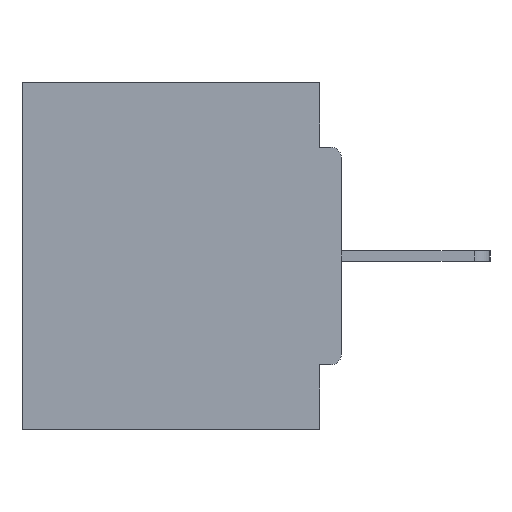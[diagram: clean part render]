
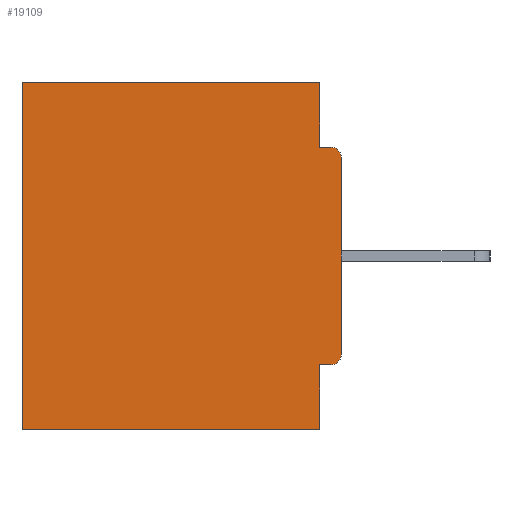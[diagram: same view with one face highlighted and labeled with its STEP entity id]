
A CAD part, left-side view. The second image highlights one B-rep face of the part: STEP entity #19109.
In plain terms, the highlighted planar face has unit normal (-1, 0, 0).
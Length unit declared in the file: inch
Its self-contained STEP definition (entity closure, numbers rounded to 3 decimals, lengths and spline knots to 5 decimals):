
#626 = LINE ( 'NONE', #946, #13052 ) ;
#946 = CARTESIAN_POINT ( 'NONE',  ( 0.298, 0., -0.5 ) ) ;
#1555 = CARTESIAN_POINT ( 'NONE',  ( 0.298, 0.46, -0.5 ) ) ;
#1739 = ORIENTED_EDGE ( 'NONE', *, *, #12474, .F. ) ;
#1782 = PLANE ( 'NONE',  #11321 ) ;
#1858 = VERTEX_POINT ( 'NONE', #20649 ) ;
#3853 = VERTEX_POINT ( 'NONE', #4302 ) ;
#4302 = CARTESIAN_POINT ( 'NONE',  ( 0.298, 0.015, -0.4065 ) ) ;
#4557 = DIRECTION ( 'NONE',  ( 0., 0., -1. ) ) ;
#5149 = VERTEX_POINT ( 'NONE', #24113 ) ;
#5207 = AXIS2_PLACEMENT_3D ( 'NONE', #11761, #21563, #4557 ) ;
#5361 = CARTESIAN_POINT ( 'NONE',  ( 0.298, 0., -0.4065 ) ) ;
#5367 = EDGE_CURVE ( 'NONE', #5149, #21112, #19919, .T. ) ;
#5705 = CARTESIAN_POINT ( 'NONE',  ( 0.298, 0., 0. ) ) ;
#8097 = CIRCLE ( 'NONE', #12087, 0.015 ) ;
#8732 = CARTESIAN_POINT ( 'NONE',  ( 0.298, 0., -0.1085 ) ) ;
#9196 = VERTEX_POINT ( 'NONE', #18671 ) ;
#9324 = VERTEX_POINT ( 'NONE', #21785 ) ;
#9512 = CARTESIAN_POINT ( 'NONE',  ( 0.298, 0., -0.0935 ) ) ;
#10154 = DIRECTION ( 'NONE',  ( 0., 0., -1. ) ) ;
#11321 = AXIS2_PLACEMENT_3D ( 'NONE', #25794, #23452, #14273 ) ;
#11423 = EDGE_LOOP ( 'NONE', ( #27357, #12553, #22717, #27432, #28200, #18903, #1739, #23394, #21297, #25021 ) ) ;
#11467 = EDGE_CURVE ( 'NONE', #22244, #21112, #626, .T. ) ;
#11478 = LINE ( 'NONE', #13827, #24116 ) ;
#11616 = VECTOR ( 'NONE', #10154, 39.37008 ) ;
#11761 = CARTESIAN_POINT ( 'NONE',  ( 0.298, 0.015, -0.1085 ) ) ;
#12087 = AXIS2_PLACEMENT_3D ( 'NONE', #19408, #28890, #16598 ) ;
#12359 = LINE ( 'NONE', #26684, #11616 ) ;
#12474 = EDGE_CURVE ( 'NONE', #9196, #22244, #12359, .T. ) ;
#12553 = ORIENTED_EDGE ( 'NONE', *, *, #28737, .F. ) ;
#12745 = LINE ( 'NONE', #5705, #22234 ) ;
#13052 = VECTOR ( 'NONE', #29310, 39.37008 ) ;
#13217 = DIRECTION ( 'NONE',  ( 0., 0., -1. ) ) ;
#13627 = EDGE_CURVE ( 'NONE', #9324, #1858, #11478, .T. ) ;
#13827 = CARTESIAN_POINT ( 'NONE',  ( 0.298, 0.031, -0.5 ) ) ;
#14273 = DIRECTION ( 'NONE',  ( 0., 0., -1. ) ) ;
#14482 = VERTEX_POINT ( 'NONE', #17822 ) ;
#15047 = VERTEX_POINT ( 'NONE', #8732 ) ;
#15240 = DIRECTION ( 'NONE',  ( 0., 0., -1. ) ) ;
#15857 = CARTESIAN_POINT ( 'NONE',  ( 0.298, 0.46, 0. ) ) ;
#16598 = DIRECTION ( 'NONE',  ( 0., 0., -1. ) ) ;
#16699 = CARTESIAN_POINT ( 'NONE',  ( 0.298, 0., 0. ) ) ;
#17670 = LINE ( 'NONE', #5361, #30646 ) ;
#17822 = CARTESIAN_POINT ( 'NONE',  ( 0.298, 0.015, -0.0935 ) ) ;
#18617 = VECTOR ( 'NONE', #30551, 39.37008 ) ;
#18671 = CARTESIAN_POINT ( 'NONE',  ( 0.298, 0.031, -0.4065 ) ) ;
#18903 = ORIENTED_EDGE ( 'NONE', *, *, #11467, .F. ) ;
#19109 = ADVANCED_FACE ( 'NONE', ( #25640 ), #1782, .F. ) ;
#19204 = LINE ( 'NONE', #16699, #20735 ) ;
#19408 = CARTESIAN_POINT ( 'NONE',  ( 0.298, 0.015, -0.3915 ) ) ;
#19919 = LINE ( 'NONE', #15857, #24132 ) ;
#20649 = CARTESIAN_POINT ( 'NONE',  ( 0.298, 0.031, -0.0935 ) ) ;
#20712 = VERTEX_POINT ( 'NONE', #28084 ) ;
#20735 = VECTOR ( 'NONE', #28701, 39.37008 ) ;
#21112 = VERTEX_POINT ( 'NONE', #1555 ) ;
#21297 = ORIENTED_EDGE ( 'NONE', *, *, #26531, .T. ) ;
#21563 = DIRECTION ( 'NONE',  ( -1., 0., 0. ) ) ;
#21682 = LINE ( 'NONE', #9512, #18617 ) ;
#21785 = CARTESIAN_POINT ( 'NONE',  ( 0.298, 0.031, 0. ) ) ;
#22234 = VECTOR ( 'NONE', #15240, 39.37008 ) ;
#22244 = VERTEX_POINT ( 'NONE', #29163 ) ;
#22717 = ORIENTED_EDGE ( 'NONE', *, *, #13627, .F. ) ;
#23394 = ORIENTED_EDGE ( 'NONE', *, *, #23494, .F. ) ;
#23452 = DIRECTION ( 'NONE',  ( 1., 0., 0. ) ) ;
#23494 = EDGE_CURVE ( 'NONE', #3853, #9196, #17670, .T. ) ;
#24113 = CARTESIAN_POINT ( 'NONE',  ( 0.298, 0.46, 0. ) ) ;
#24116 = VECTOR ( 'NONE', #28138, 39.37008 ) ;
#24132 = VECTOR ( 'NONE', #13217, 39.37008 ) ;
#24366 = DIRECTION ( 'NONE',  ( 0., 1., 0. ) ) ;
#25021 = ORIENTED_EDGE ( 'NONE', *, *, #26083, .F. ) ;
#25640 = FACE_OUTER_BOUND ( 'NONE', #11423, .T. ) ;
#25794 = CARTESIAN_POINT ( 'NONE',  ( 0.298, 0., 0. ) ) ;
#26083 = EDGE_CURVE ( 'NONE', #15047, #20712, #12745, .T. ) ;
#26531 = EDGE_CURVE ( 'NONE', #3853, #20712, #8097, .T. ) ;
#26684 = CARTESIAN_POINT ( 'NONE',  ( 0.298, 0.031, -0.5 ) ) ;
#27104 = CIRCLE ( 'NONE', #5207, 0.015 ) ;
#27357 = ORIENTED_EDGE ( 'NONE', *, *, #29464, .T. ) ;
#27432 = ORIENTED_EDGE ( 'NONE', *, *, #30326, .T. ) ;
#28084 = CARTESIAN_POINT ( 'NONE',  ( 0.298, 0., -0.3915 ) ) ;
#28138 = DIRECTION ( 'NONE',  ( 0., 0., -1. ) ) ;
#28200 = ORIENTED_EDGE ( 'NONE', *, *, #5367, .T. ) ;
#28701 = DIRECTION ( 'NONE',  ( 0., 1., 0. ) ) ;
#28737 = EDGE_CURVE ( 'NONE', #1858, #14482, #21682, .T. ) ;
#28890 = DIRECTION ( 'NONE',  ( -1., 0., 0. ) ) ;
#29163 = CARTESIAN_POINT ( 'NONE',  ( 0.298, 0.031, -0.5 ) ) ;
#29310 = DIRECTION ( 'NONE',  ( 0., 1., 0. ) ) ;
#29464 = EDGE_CURVE ( 'NONE', #15047, #14482, #27104, .T. ) ;
#30326 = EDGE_CURVE ( 'NONE', #9324, #5149, #19204, .T. ) ;
#30551 = DIRECTION ( 'NONE',  ( 0., -1., 0. ) ) ;
#30646 = VECTOR ( 'NONE', #24366, 39.37008 ) ;
